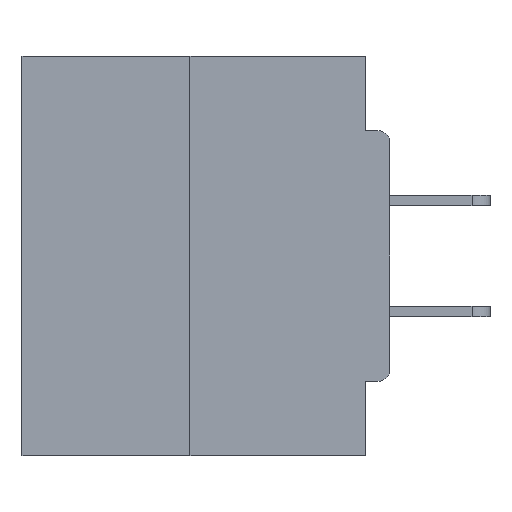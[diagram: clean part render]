
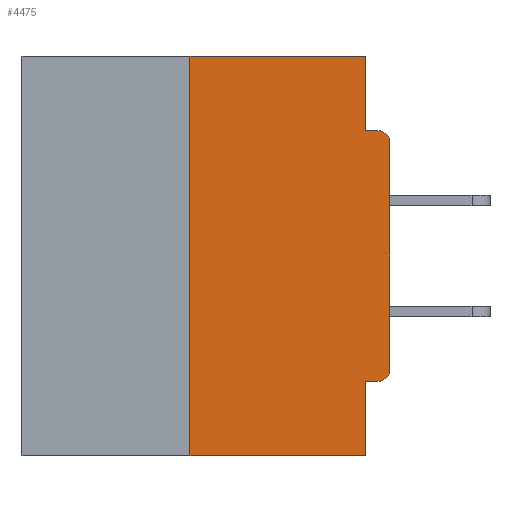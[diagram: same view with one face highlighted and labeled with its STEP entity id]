
A CAD part, left-side view. The second image highlights one B-rep face of the part: STEP entity #4475.
In plain terms, the highlighted planar face has unit normal (-1, 0, 0).
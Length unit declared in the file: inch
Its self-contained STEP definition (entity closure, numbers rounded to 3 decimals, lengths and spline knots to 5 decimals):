
#411 = DIRECTION ( 'NONE',  ( -1., 0., 0. ) ) ;
#630 = CARTESIAN_POINT ( 'NONE',  ( 0., 0.46, 0. ) ) ;
#1601 = FACE_OUTER_BOUND ( 'NONE', #30200, .T. ) ;
#2025 = LINE ( 'NONE', #20985, #6026 ) ;
#2398 = VECTOR ( 'NONE', #24366, 39.37008 ) ;
#2973 = ORIENTED_EDGE ( 'NONE', *, *, #30747, .F. ) ;
#3111 = DIRECTION ( 'NONE',  ( 0., -1., 0. ) ) ;
#3598 = VERTEX_POINT ( 'NONE', #32998 ) ;
#3719 = LINE ( 'NONE', #7064, #2398 ) ;
#3808 = EDGE_CURVE ( 'NONE', #32307, #9093, #28492, .T. ) ;
#4475 = ADVANCED_FACE ( 'NONE', ( #1601 ), #9045, .F. ) ;
#4707 = VERTEX_POINT ( 'NONE', #10610 ) ;
#5107 = ORIENTED_EDGE ( 'NONE', *, *, #34136, .T. ) ;
#5337 = ORIENTED_EDGE ( 'NONE', *, *, #13872, .T. ) ;
#6026 = VECTOR ( 'NONE', #26765, 39.37008 ) ;
#6870 = VECTOR ( 'NONE', #9499, 39.37008 ) ;
#7064 = CARTESIAN_POINT ( 'NONE',  ( 0., 0., -0.4065 ) ) ;
#7623 = DIRECTION ( 'NONE',  ( 0., 0., 1. ) ) ;
#7700 = CARTESIAN_POINT ( 'NONE',  ( 0., 0.031, -0.0935 ) ) ;
#8763 = VERTEX_POINT ( 'NONE', #28937 ) ;
#8924 = DIRECTION ( 'NONE',  ( 1., 0., 0. ) ) ;
#9045 = PLANE ( 'NONE',  #26662 ) ;
#9093 = VERTEX_POINT ( 'NONE', #9174 ) ;
#9174 = CARTESIAN_POINT ( 'NONE',  ( 0., 0.031, -0.5 ) ) ;
#9370 = DIRECTION ( 'NONE',  ( 0., 0., -1. ) ) ;
#9499 = DIRECTION ( 'NONE',  ( 0., 0., 1. ) ) ;
#10610 = CARTESIAN_POINT ( 'NONE',  ( 0., 0.015, -0.4065 ) ) ;
#10626 = VECTOR ( 'NONE', #25910, 39.37008 ) ;
#13057 = CARTESIAN_POINT ( 'NONE',  ( 0., 0.46, -0.5 ) ) ;
#13473 = ORIENTED_EDGE ( 'NONE', *, *, #31963, .F. ) ;
#13872 = EDGE_CURVE ( 'NONE', #4707, #8763, #36100, .T. ) ;
#15045 = CARTESIAN_POINT ( 'NONE',  ( 0., 0., 0. ) ) ;
#16316 = LINE ( 'NONE', #630, #25750 ) ;
#16426 = ORIENTED_EDGE ( 'NONE', *, *, #3808, .T. ) ;
#17246 = CARTESIAN_POINT ( 'NONE',  ( 0., 0.031, 0. ) ) ;
#17539 = DIRECTION ( 'NONE',  ( 0., 0., -1. ) ) ;
#17575 = VERTEX_POINT ( 'NONE', #36172 ) ;
#17708 = VERTEX_POINT ( 'NONE', #27937 ) ;
#17733 = DIRECTION ( 'NONE',  ( 0., 0., -1. ) ) ;
#17863 = ORIENTED_EDGE ( 'NONE', *, *, #28035, .F. ) ;
#18009 = CARTESIAN_POINT ( 'NONE',  ( 0., 0.25, 0. ) ) ;
#18376 = VECTOR ( 'NONE', #32462, 39.37008 ) ;
#18959 = VERTEX_POINT ( 'NONE', #28818 ) ;
#20084 = EDGE_CURVE ( 'NONE', #3598, #34771, #20521, .T. ) ;
#20521 = LINE ( 'NONE', #17246, #10626 ) ;
#20671 = ORIENTED_EDGE ( 'NONE', *, *, #20084, .F. ) ;
#20796 = CARTESIAN_POINT ( 'NONE',  ( 0., 0.015, -0.1085 ) ) ;
#20985 = CARTESIAN_POINT ( 'NONE',  ( 0., 0., -0.0935 ) ) ;
#21782 = VERTEX_POINT ( 'NONE', #18009 ) ;
#21815 = ORIENTED_EDGE ( 'NONE', *, *, #36787, .F. ) ;
#23647 = CARTESIAN_POINT ( 'NONE',  ( 0., 0.031, -0.5 ) ) ;
#24324 = AXIS2_PLACEMENT_3D ( 'NONE', #20796, #411, #9370 ) ;
#24366 = DIRECTION ( 'NONE',  ( 0., 1., 0. ) ) ;
#24421 = VECTOR ( 'NONE', #24675, 39.37008 ) ;
#24675 = DIRECTION ( 'NONE',  ( 0., -1., 0. ) ) ;
#25721 = CARTESIAN_POINT ( 'NONE',  ( 0., 0.46, 0. ) ) ;
#25750 = VECTOR ( 'NONE', #3111, 39.37008 ) ;
#25910 = DIRECTION ( 'NONE',  ( 0., 0., -1. ) ) ;
#26361 = CARTESIAN_POINT ( 'NONE',  ( 0., 0.25, -0.5 ) ) ;
#26662 = AXIS2_PLACEMENT_3D ( 'NONE', #25721, #8924, #17539 ) ;
#26765 = DIRECTION ( 'NONE',  ( 0., -1., 0. ) ) ;
#26786 = VECTOR ( 'NONE', #7623, 39.37008 ) ;
#27689 = LINE ( 'NONE', #33124, #26786 ) ;
#27937 = CARTESIAN_POINT ( 'NONE',  ( 0., 0.015, -0.0935 ) ) ;
#28035 = EDGE_CURVE ( 'NONE', #21782, #3598, #16316, .T. ) ;
#28492 = LINE ( 'NONE', #13057, #24421 ) ;
#28761 = LINE ( 'NONE', #23647, #18376 ) ;
#28818 = CARTESIAN_POINT ( 'NONE',  ( 0., 0., -0.1085 ) ) ;
#28937 = CARTESIAN_POINT ( 'NONE',  ( 0., 0., -0.3915 ) ) ;
#29169 = EDGE_CURVE ( 'NONE', #8763, #18959, #32492, .T. ) ;
#30200 = EDGE_LOOP ( 'NONE', ( #17863, #32439, #16426, #2973, #13473, #5337, #35624, #5107, #21815, #20671 ) ) ;
#30747 = EDGE_CURVE ( 'NONE', #17575, #9093, #28761, .T. ) ;
#31238 = AXIS2_PLACEMENT_3D ( 'NONE', #32350, #32093, #17733 ) ;
#31963 = EDGE_CURVE ( 'NONE', #4707, #17575, #3719, .T. ) ;
#32093 = DIRECTION ( 'NONE',  ( -1., 0., 0. ) ) ;
#32307 = VERTEX_POINT ( 'NONE', #26361 ) ;
#32350 = CARTESIAN_POINT ( 'NONE',  ( 0., 0.015, -0.3915 ) ) ;
#32439 = ORIENTED_EDGE ( 'NONE', *, *, #35701, .F. ) ;
#32462 = DIRECTION ( 'NONE',  ( 0., 0., -1. ) ) ;
#32492 = LINE ( 'NONE', #15045, #6870 ) ;
#32998 = CARTESIAN_POINT ( 'NONE',  ( 0., 0.031, 0. ) ) ;
#33124 = CARTESIAN_POINT ( 'NONE',  ( 0., 0.25, 0. ) ) ;
#34136 = EDGE_CURVE ( 'NONE', #18959, #17708, #35864, .T. ) ;
#34771 = VERTEX_POINT ( 'NONE', #7700 ) ;
#35624 = ORIENTED_EDGE ( 'NONE', *, *, #29169, .T. ) ;
#35701 = EDGE_CURVE ( 'NONE', #32307, #21782, #27689, .T. ) ;
#35864 = CIRCLE ( 'NONE', #24324, 0.015 ) ;
#36100 = CIRCLE ( 'NONE', #31238, 0.015 ) ;
#36172 = CARTESIAN_POINT ( 'NONE',  ( 0., 0.031, -0.4065 ) ) ;
#36787 = EDGE_CURVE ( 'NONE', #34771, #17708, #2025, .T. ) ;
